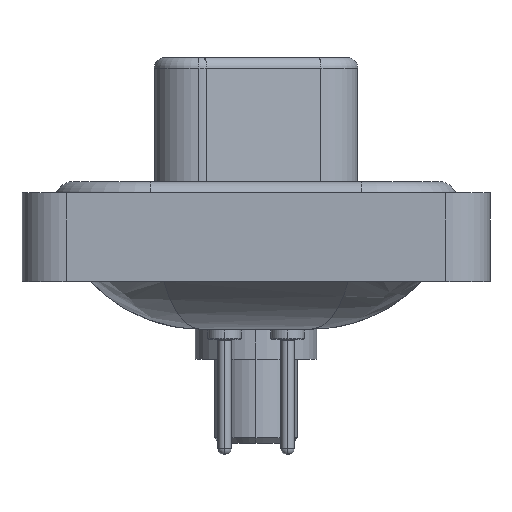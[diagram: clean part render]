
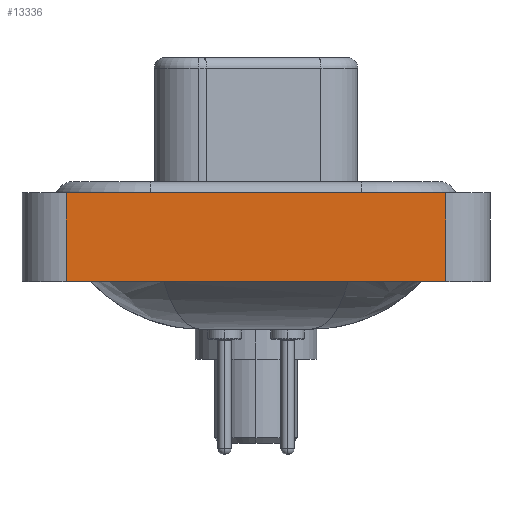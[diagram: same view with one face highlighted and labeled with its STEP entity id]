
A CAD part, left-side view. The second image highlights one B-rep face of the part: STEP entity #13336.
In plain terms, the highlighted planar face has unit normal (-1, 0, 0).
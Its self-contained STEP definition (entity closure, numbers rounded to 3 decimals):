
#1640 = EDGE_CURVE ( 'NONE', #4714, #23932, #16235, .T. ) ;
#1985 = CARTESIAN_POINT ( 'NONE',  ( -7.35, -8.55, 0.4 ) ) ;
#2346 = CARTESIAN_POINT ( 'NONE',  ( -7.35, 8.55, 0.4 ) ) ;
#2357 = EDGE_CURVE ( 'NONE', #21118, #7972, #6292, .T. ) ;
#2774 = DIRECTION ( 'NONE',  ( 0., -1., 0. ) ) ;
#4292 = CARTESIAN_POINT ( 'NONE',  ( -7.35, 8.55, -3.6 ) ) ;
#4714 = VERTEX_POINT ( 'NONE', #21669 ) ;
#4830 = PLANE ( 'NONE',  #10272 ) ;
#4914 = ORIENTED_EDGE ( 'NONE', *, *, #11868, .T. ) ;
#5115 = CARTESIAN_POINT ( 'NONE',  ( -7.35, -8.55, -3.6 ) ) ;
#6292 = LINE ( 'NONE', #1985, #18674 ) ;
#7912 = DIRECTION ( 'NONE',  ( 0., -1., 0. ) ) ;
#7972 = VERTEX_POINT ( 'NONE', #8723 ) ;
#8723 = CARTESIAN_POINT ( 'NONE',  ( -7.35, -8.55, 0.4 ) ) ;
#9746 = VECTOR ( 'NONE', #20985, 1000. ) ;
#10021 = DIRECTION ( 'NONE',  ( -1., 0., 0. ) ) ;
#10181 = ORIENTED_EDGE ( 'NONE', *, *, #2357, .F. ) ;
#10272 = AXIS2_PLACEMENT_3D ( 'NONE', #23120, #10021, #19900 ) ;
#10779 = LINE ( 'NONE', #21896, #18458 ) ;
#11748 = EDGE_CURVE ( 'NONE', #4714, #21118, #13460, .T. ) ;
#11868 = EDGE_CURVE ( 'NONE', #23932, #7972, #10779, .T. ) ;
#12189 = ORIENTED_EDGE ( 'NONE', *, *, #11748, .F. ) ;
#12885 = DIRECTION ( 'NONE',  ( 0., 0., 1. ) ) ;
#13336 = ADVANCED_FACE ( 'NONE', ( #16068 ), #4830, .T. ) ;
#13460 = LINE ( 'NONE', #4292, #9746 ) ;
#16068 = FACE_OUTER_BOUND ( 'NONE', #17958, .T. ) ;
#16235 = LINE ( 'NONE', #5115, #16674 ) ;
#16474 = CARTESIAN_POINT ( 'NONE',  ( -7.35, -8.55, -3.6 ) ) ;
#16674 = VECTOR ( 'NONE', #2774, 1000. ) ;
#17958 = EDGE_LOOP ( 'NONE', ( #4914, #10181, #12189, #22531 ) ) ;
#18458 = VECTOR ( 'NONE', #12885, 1000. ) ;
#18674 = VECTOR ( 'NONE', #7912, 1000. ) ;
#19900 = DIRECTION ( 'NONE',  ( 0., 0., 1. ) ) ;
#20985 = DIRECTION ( 'NONE',  ( 0., 0., 1. ) ) ;
#21118 = VERTEX_POINT ( 'NONE', #2346 ) ;
#21669 = CARTESIAN_POINT ( 'NONE',  ( -7.35, 8.55, -3.6 ) ) ;
#21896 = CARTESIAN_POINT ( 'NONE',  ( -7.35, -8.55, -3.6 ) ) ;
#22531 = ORIENTED_EDGE ( 'NONE', *, *, #1640, .T. ) ;
#23120 = CARTESIAN_POINT ( 'NONE',  ( -7.35, -8.55, -3.6 ) ) ;
#23932 = VERTEX_POINT ( 'NONE', #16474 ) ;
